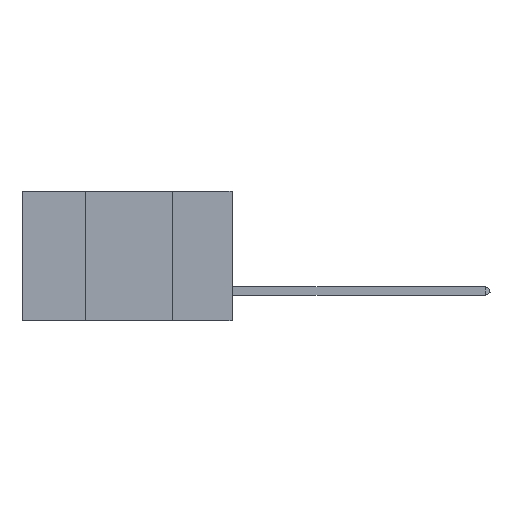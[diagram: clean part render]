
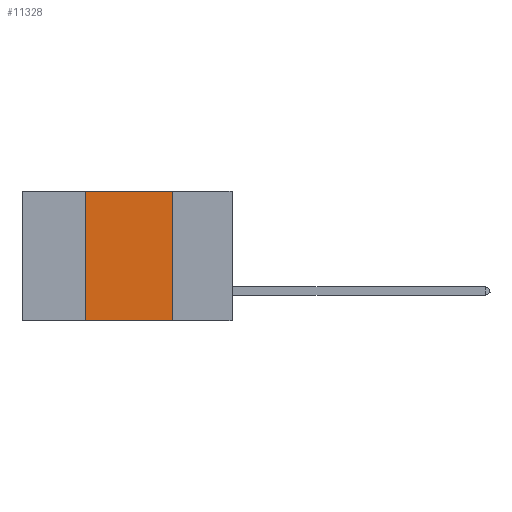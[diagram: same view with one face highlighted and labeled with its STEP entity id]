
A CAD part, left-side view. The second image highlights one B-rep face of the part: STEP entity #11328.
In plain terms, the highlighted planar face has unit normal (-1, 0, 0).
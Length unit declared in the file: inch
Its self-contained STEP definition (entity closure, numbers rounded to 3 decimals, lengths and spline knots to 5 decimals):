
#357 = DIRECTION ( 'NONE',  ( 0., 0., -1. ) ) ;
#1645 = CARTESIAN_POINT ( 'NONE',  ( 0., 0.6, -0.37 ) ) ;
#2095 = EDGE_CURVE ( 'NONE', #3366, #2641, #10543, .T. ) ;
#2292 = LINE ( 'NONE', #1645, #7942 ) ;
#2641 = VERTEX_POINT ( 'NONE', #15016 ) ;
#2921 = LINE ( 'NONE', #12263, #11419 ) ;
#3055 = ORIENTED_EDGE ( 'NONE', *, *, #9363, .F. ) ;
#3366 = VERTEX_POINT ( 'NONE', #18064 ) ;
#3955 = CARTESIAN_POINT ( 'NONE',  ( 0., 0.42, 0. ) ) ;
#4645 = VERTEX_POINT ( 'NONE', #16691 ) ;
#5212 = FACE_OUTER_BOUND ( 'NONE', #8682, .T. ) ;
#5558 = ORIENTED_EDGE ( 'NONE', *, *, #13566, .T. ) ;
#5775 = VERTEX_POINT ( 'NONE', #13962 ) ;
#6643 = DIRECTION ( 'NONE',  ( 0., 0., 1. ) ) ;
#6797 = LINE ( 'NONE', #3955, #17531 ) ;
#7429 = AXIS2_PLACEMENT_3D ( 'NONE', #17103, #10089, #357 ) ;
#7776 = CARTESIAN_POINT ( 'NONE',  ( 0., 0.17, 0. ) ) ;
#7942 = VECTOR ( 'NONE', #17127, 39.37008 ) ;
#7994 = EDGE_CURVE ( 'NONE', #4645, #3366, #2921, .T. ) ;
#8202 = ORIENTED_EDGE ( 'NONE', *, *, #7994, .F. ) ;
#8682 = EDGE_LOOP ( 'NONE', ( #12757, #8202, #3055, #5558 ) ) ;
#9363 = EDGE_CURVE ( 'NONE', #5775, #4645, #6797, .T. ) ;
#10089 = DIRECTION ( 'NONE',  ( 1., 0., 0. ) ) ;
#10543 = LINE ( 'NONE', #7776, #17580 ) ;
#11328 = ADVANCED_FACE ( 'NONE', ( #5212 ), #11388, .F. ) ;
#11388 = PLANE ( 'NONE',  #7429 ) ;
#11419 = VECTOR ( 'NONE', #12323, 39.37008 ) ;
#11757 = DIRECTION ( 'NONE',  ( 0., 0., -1. ) ) ;
#12263 = CARTESIAN_POINT ( 'NONE',  ( 0., 0.6, 0. ) ) ;
#12323 = DIRECTION ( 'NONE',  ( 0., -1., 0. ) ) ;
#12757 = ORIENTED_EDGE ( 'NONE', *, *, #2095, .F. ) ;
#13566 = EDGE_CURVE ( 'NONE', #5775, #2641, #2292, .T. ) ;
#13962 = CARTESIAN_POINT ( 'NONE',  ( 0., 0.42, -0.37 ) ) ;
#15016 = CARTESIAN_POINT ( 'NONE',  ( 0., 0.17, -0.37 ) ) ;
#16691 = CARTESIAN_POINT ( 'NONE',  ( 0., 0.42, 0. ) ) ;
#17103 = CARTESIAN_POINT ( 'NONE',  ( 0., 0.6, 0. ) ) ;
#17127 = DIRECTION ( 'NONE',  ( 0., -1., 0. ) ) ;
#17531 = VECTOR ( 'NONE', #6643, 39.37008 ) ;
#17580 = VECTOR ( 'NONE', #11757, 39.37008 ) ;
#18064 = CARTESIAN_POINT ( 'NONE',  ( 0., 0.17, 0. ) ) ;
